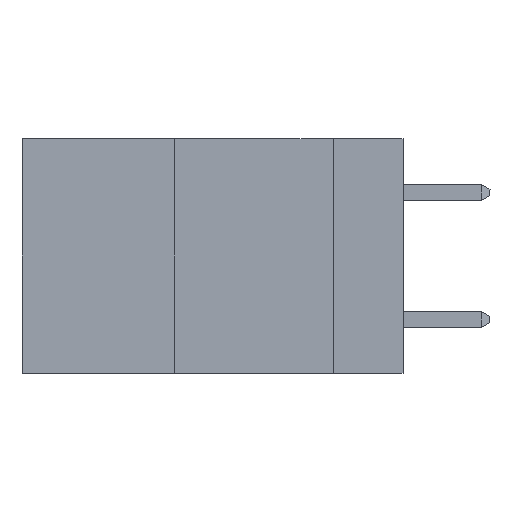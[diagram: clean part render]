
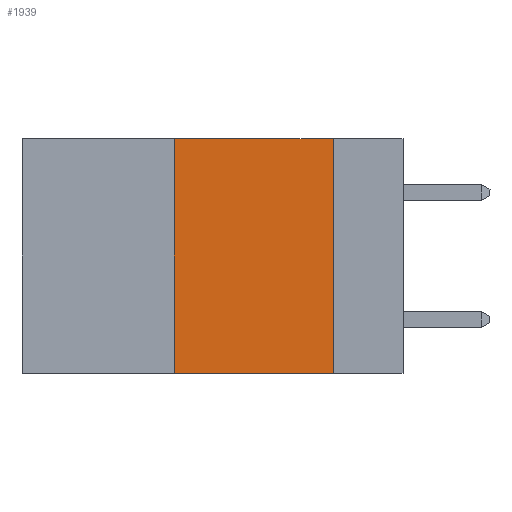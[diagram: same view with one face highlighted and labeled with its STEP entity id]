
A CAD part, left-side view. The second image highlights one B-rep face of the part: STEP entity #1939.
In plain terms, the highlighted planar face has unit normal (-1, 0, 0).
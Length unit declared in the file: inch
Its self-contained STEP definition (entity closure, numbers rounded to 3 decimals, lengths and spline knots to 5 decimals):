
#497 = CARTESIAN_POINT ( 'NONE',  ( 0., 0.6, 0. ) ) ;
#1939 = ADVANCED_FACE ( 'NONE', ( #2879 ), #6826, .F. ) ;
#2026 = CARTESIAN_POINT ( 'NONE',  ( 0., 0.6, 0. ) ) ;
#2433 = VERTEX_POINT ( 'NONE', #4111 ) ;
#2445 = VECTOR ( 'NONE', #4192, 39.37008 ) ;
#2601 = ORIENTED_EDGE ( 'NONE', *, *, #3177, .T. ) ;
#2607 = CARTESIAN_POINT ( 'NONE',  ( 0., 0.11, 0. ) ) ;
#2879 = FACE_OUTER_BOUND ( 'NONE', #3291, .T. ) ;
#3119 = DIRECTION ( 'NONE',  ( 0., -1., 0. ) ) ;
#3177 = EDGE_CURVE ( 'NONE', #2433, #4556, #5272, .T. ) ;
#3181 = DIRECTION ( 'NONE',  ( 0., 0., -1. ) ) ;
#3291 = EDGE_LOOP ( 'NONE', ( #10501, #8705, #6833, #2601 ) ) ;
#4111 = CARTESIAN_POINT ( 'NONE',  ( 0., 0.36, -0.37 ) ) ;
#4192 = DIRECTION ( 'NONE',  ( 0., -1., 0. ) ) ;
#4556 = VERTEX_POINT ( 'NONE', #6361 ) ;
#4578 = DIRECTION ( 'NONE',  ( 0., 0., 1. ) ) ;
#4798 = VECTOR ( 'NONE', #6544, 39.37008 ) ;
#4956 = LINE ( 'NONE', #497, #2445 ) ;
#5272 = LINE ( 'NONE', #6240, #9588 ) ;
#6134 = AXIS2_PLACEMENT_3D ( 'NONE', #2026, #8262, #3181 ) ;
#6240 = CARTESIAN_POINT ( 'NONE',  ( 0., 0.6, -0.37 ) ) ;
#6361 = CARTESIAN_POINT ( 'NONE',  ( 0., 0.11, -0.37 ) ) ;
#6544 = DIRECTION ( 'NONE',  ( 0., 0., -1. ) ) ;
#6826 = PLANE ( 'NONE',  #6134 ) ;
#6833 = ORIENTED_EDGE ( 'NONE', *, *, #8340, .F. ) ;
#7929 = CARTESIAN_POINT ( 'NONE',  ( 0., 0.36, 0. ) ) ;
#8262 = DIRECTION ( 'NONE',  ( 1., 0., 0. ) ) ;
#8307 = VERTEX_POINT ( 'NONE', #2607 ) ;
#8340 = EDGE_CURVE ( 'NONE', #2433, #10718, #10981, .T. ) ;
#8705 = ORIENTED_EDGE ( 'NONE', *, *, #8903, .F. ) ;
#8903 = EDGE_CURVE ( 'NONE', #10718, #8307, #4956, .T. ) ;
#8921 = CARTESIAN_POINT ( 'NONE',  ( 0., 0.11, 0. ) ) ;
#8940 = VECTOR ( 'NONE', #4578, 39.37008 ) ;
#9151 = LINE ( 'NONE', #8921, #4798 ) ;
#9588 = VECTOR ( 'NONE', #3119, 39.37008 ) ;
#10091 = EDGE_CURVE ( 'NONE', #8307, #4556, #9151, .T. ) ;
#10501 = ORIENTED_EDGE ( 'NONE', *, *, #10091, .F. ) ;
#10718 = VERTEX_POINT ( 'NONE', #11024 ) ;
#10981 = LINE ( 'NONE', #7929, #8940 ) ;
#11024 = CARTESIAN_POINT ( 'NONE',  ( 0., 0.36, 0. ) ) ;
